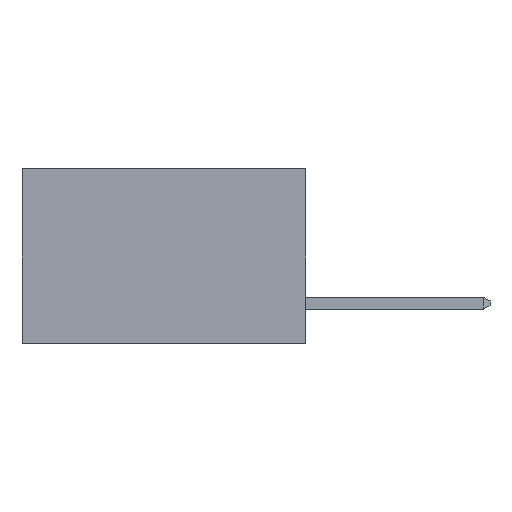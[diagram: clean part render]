
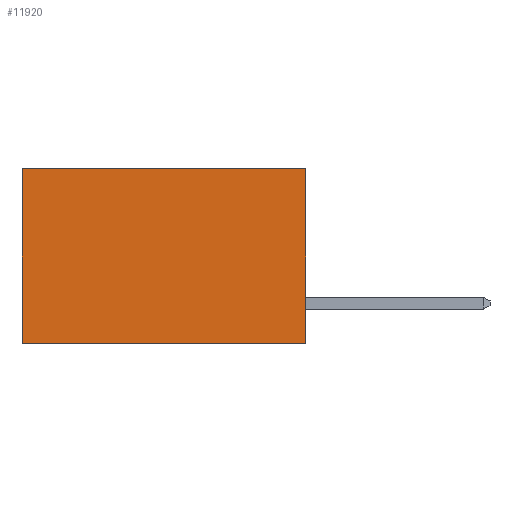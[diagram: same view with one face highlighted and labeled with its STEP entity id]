
A CAD part, left-side view. The second image highlights one B-rep face of the part: STEP entity #11920.
In plain terms, the highlighted planar face has unit normal (-1, 0, 0).
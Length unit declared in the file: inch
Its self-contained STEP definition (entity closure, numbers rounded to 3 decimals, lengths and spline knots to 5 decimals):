
#233 = VERTEX_POINT ( 'NONE', #11564 ) ;
#240 = EDGE_CURVE ( 'NONE', #12819, #9832, #3041, .T. ) ;
#272 = LINE ( 'NONE', #6346, #9342 ) ;
#627 = VECTOR ( 'NONE', #7531, 39.37008 ) ;
#788 = DIRECTION ( 'NONE',  ( 0., 0., -1. ) ) ;
#1112 = EDGE_CURVE ( 'NONE', #13268, #233, #272, .T. ) ;
#3041 = LINE ( 'NONE', #9498, #627 ) ;
#3398 = DIRECTION ( 'NONE',  ( 0., 0., -1. ) ) ;
#3558 = DIRECTION ( 'NONE',  ( 0., 1., 0. ) ) ;
#4751 = EDGE_CURVE ( 'NONE', #13268, #12819, #7520, .T. ) ;
#5042 = CARTESIAN_POINT ( 'NONE',  ( 0.2615, 0.6, -0.37 ) ) ;
#5330 = LINE ( 'NONE', #8938, #12919 ) ;
#5499 = CARTESIAN_POINT ( 'NONE',  ( 0.2615, 0., 0. ) ) ;
#6324 = EDGE_LOOP ( 'NONE', ( #12775, #7393, #11829, #12458 ) ) ;
#6346 = CARTESIAN_POINT ( 'NONE',  ( 0.2615, 0., -0.37 ) ) ;
#6987 = DIRECTION ( 'NONE',  ( 1., 0., 0. ) ) ;
#7393 = ORIENTED_EDGE ( 'NONE', *, *, #10333, .F. ) ;
#7520 = LINE ( 'NONE', #9584, #8505 ) ;
#7531 = DIRECTION ( 'NONE',  ( 0., 0., -1. ) ) ;
#8034 = AXIS2_PLACEMENT_3D ( 'NONE', #12125, #6987, #788 ) ;
#8505 = VECTOR ( 'NONE', #3558, 39.37008 ) ;
#8830 = CARTESIAN_POINT ( 'NONE',  ( 0.2615, 0.6, 0. ) ) ;
#8938 = CARTESIAN_POINT ( 'NONE',  ( 0.2615, 0., -0.37 ) ) ;
#9073 = PLANE ( 'NONE',  #8034 ) ;
#9342 = VECTOR ( 'NONE', #3398, 39.37008 ) ;
#9498 = CARTESIAN_POINT ( 'NONE',  ( 0.2615, 0.6, -0.37 ) ) ;
#9584 = CARTESIAN_POINT ( 'NONE',  ( 0.2615, 0., 0. ) ) ;
#9832 = VERTEX_POINT ( 'NONE', #5042 ) ;
#10027 = DIRECTION ( 'NONE',  ( 0., 1., 0. ) ) ;
#10333 = EDGE_CURVE ( 'NONE', #233, #9832, #5330, .T. ) ;
#11109 = FACE_OUTER_BOUND ( 'NONE', #6324, .T. ) ;
#11564 = CARTESIAN_POINT ( 'NONE',  ( 0.2615, 0., -0.37 ) ) ;
#11829 = ORIENTED_EDGE ( 'NONE', *, *, #1112, .F. ) ;
#11920 = ADVANCED_FACE ( 'NONE', ( #11109 ), #9073, .F. ) ;
#12125 = CARTESIAN_POINT ( 'NONE',  ( 0.2615, 0., -0.37 ) ) ;
#12458 = ORIENTED_EDGE ( 'NONE', *, *, #4751, .T. ) ;
#12775 = ORIENTED_EDGE ( 'NONE', *, *, #240, .T. ) ;
#12819 = VERTEX_POINT ( 'NONE', #8830 ) ;
#12919 = VECTOR ( 'NONE', #10027, 39.37008 ) ;
#13268 = VERTEX_POINT ( 'NONE', #5499 ) ;
